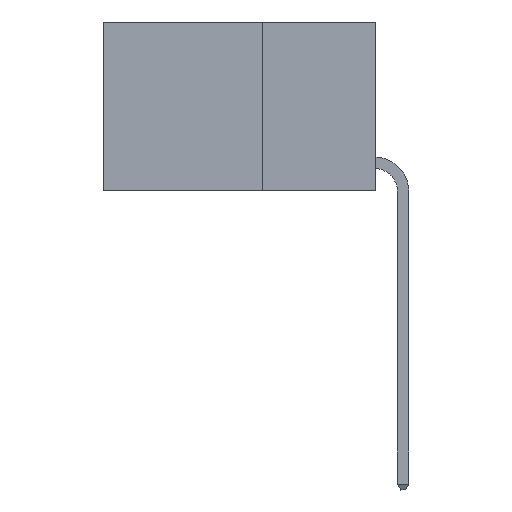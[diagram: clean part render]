
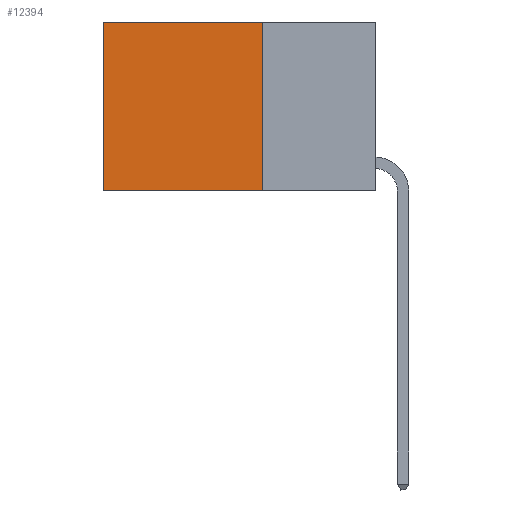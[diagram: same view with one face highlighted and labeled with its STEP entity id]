
A CAD part, left-side view. The second image highlights one B-rep face of the part: STEP entity #12394.
In plain terms, the highlighted planar face has unit normal (-1, 0, 0).
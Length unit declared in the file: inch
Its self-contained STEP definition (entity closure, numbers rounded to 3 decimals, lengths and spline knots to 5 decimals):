
#457 = CARTESIAN_POINT ( 'NONE',  ( 0.2625, 0.6, -0.37 ) ) ;
#521 = DIRECTION ( 'NONE',  ( 0., 0., -1. ) ) ;
#1057 = CARTESIAN_POINT ( 'NONE',  ( 0.2625, 0.25, -0.37 ) ) ;
#1167 = LINE ( 'NONE', #2767, #15637 ) ;
#1332 = EDGE_CURVE ( 'NONE', #9237, #9077, #17677, .T. ) ;
#2184 = PLANE ( 'NONE',  #4454 ) ;
#2381 = VECTOR ( 'NONE', #521, 39.37008 ) ;
#2767 = CARTESIAN_POINT ( 'NONE',  ( 0.2625, 0.6, 0. ) ) ;
#3911 = CARTESIAN_POINT ( 'NONE',  ( 0.2625, 0.25, 0. ) ) ;
#4454 = AXIS2_PLACEMENT_3D ( 'NONE', #5516, #12131, #10427 ) ;
#4768 = ORIENTED_EDGE ( 'NONE', *, *, #1332, .T. ) ;
#5516 = CARTESIAN_POINT ( 'NONE',  ( 0.2625, 0.25, 0. ) ) ;
#5656 = ORIENTED_EDGE ( 'NONE', *, *, #8554, .T. ) ;
#6567 = DIRECTION ( 'NONE',  ( 0., 1., 0. ) ) ;
#6611 = DIRECTION ( 'NONE',  ( 0., 1., 0. ) ) ;
#6768 = ORIENTED_EDGE ( 'NONE', *, *, #19556, .F. ) ;
#7147 = VERTEX_POINT ( 'NONE', #1057 ) ;
#8034 = CARTESIAN_POINT ( 'NONE',  ( 0.2625, 0.25, -0.37 ) ) ;
#8416 = VECTOR ( 'NONE', #6611, 39.37008 ) ;
#8554 = EDGE_CURVE ( 'NONE', #9077, #13284, #1167, .T. ) ;
#8714 = FACE_OUTER_BOUND ( 'NONE', #21205, .T. ) ;
#9077 = VERTEX_POINT ( 'NONE', #12891 ) ;
#9237 = VERTEX_POINT ( 'NONE', #3911 ) ;
#9481 = CARTESIAN_POINT ( 'NONE',  ( 0.2625, 0.25, 0. ) ) ;
#10427 = DIRECTION ( 'NONE',  ( 0., 0., -1. ) ) ;
#12131 = DIRECTION ( 'NONE',  ( 1., 0., 0. ) ) ;
#12394 = ADVANCED_FACE ( 'NONE', ( #8714 ), #2184, .F. ) ;
#12891 = CARTESIAN_POINT ( 'NONE',  ( 0.2625, 0.6, 0. ) ) ;
#13284 = VERTEX_POINT ( 'NONE', #457 ) ;
#15028 = VECTOR ( 'NONE', #6567, 39.37008 ) ;
#15617 = ORIENTED_EDGE ( 'NONE', *, *, #20537, .F. ) ;
#15637 = VECTOR ( 'NONE', #17373, 39.37008 ) ;
#16711 = LINE ( 'NONE', #19651, #2381 ) ;
#17373 = DIRECTION ( 'NONE',  ( 0., 0., -1. ) ) ;
#17677 = LINE ( 'NONE', #9481, #8416 ) ;
#19556 = EDGE_CURVE ( 'NONE', #7147, #13284, #19700, .T. ) ;
#19651 = CARTESIAN_POINT ( 'NONE',  ( 0.2625, 0.25, 0. ) ) ;
#19700 = LINE ( 'NONE', #8034, #15028 ) ;
#20537 = EDGE_CURVE ( 'NONE', #9237, #7147, #16711, .T. ) ;
#21205 = EDGE_LOOP ( 'NONE', ( #5656, #6768, #15617, #4768 ) ) ;
